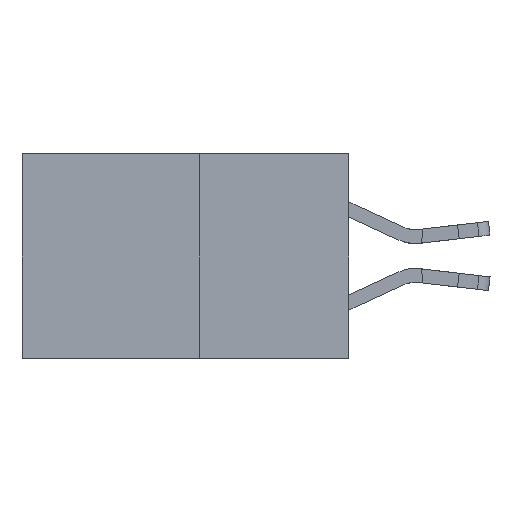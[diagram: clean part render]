
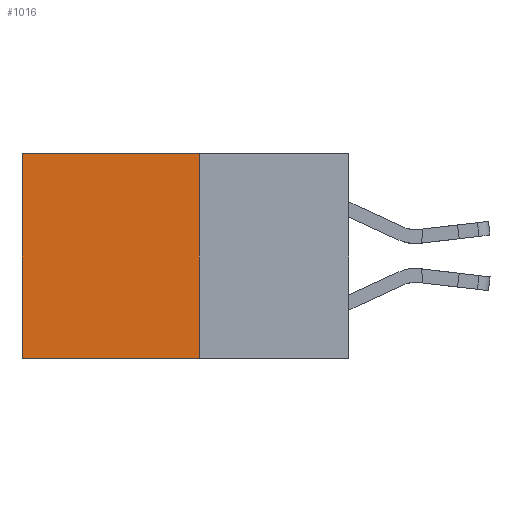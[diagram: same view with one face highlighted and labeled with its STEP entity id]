
A CAD part, left-side view. The second image highlights one B-rep face of the part: STEP entity #1016.
In plain terms, the highlighted planar face has unit normal (-1, 0, 0).
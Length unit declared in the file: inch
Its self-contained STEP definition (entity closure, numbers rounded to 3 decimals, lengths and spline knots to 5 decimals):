
#75 = VERTEX_POINT ( 'NONE', #10894 ) ;
#809 = EDGE_LOOP ( 'NONE', ( #30463, #26506, #1906, #20530 ) ) ;
#1016 = ADVANCED_FACE ( 'NONE', ( #1435 ), #16280, .F. ) ;
#1435 = FACE_OUTER_BOUND ( 'NONE', #809, .T. ) ;
#1906 = ORIENTED_EDGE ( 'NONE', *, *, #9194, .F. ) ;
#3825 = EDGE_CURVE ( 'NONE', #23485, #16942, #8904, .T. ) ;
#4219 = VECTOR ( 'NONE', #25437, 39.37008 ) ;
#5227 = DIRECTION ( 'NONE',  ( 0., 0., -1. ) ) ;
#6414 = AXIS2_PLACEMENT_3D ( 'NONE', #10796, #13680, #19462 ) ;
#8306 = CARTESIAN_POINT ( 'NONE',  ( 0.277, 0.27, -0.37 ) ) ;
#8904 = LINE ( 'NONE', #30610, #9682 ) ;
#9194 = EDGE_CURVE ( 'NONE', #11147, #75, #24392, .T. ) ;
#9682 = VECTOR ( 'NONE', #11408, 39.37008 ) ;
#10059 = LINE ( 'NONE', #8306, #4219 ) ;
#10796 = CARTESIAN_POINT ( 'NONE',  ( 0.277, 0.27, -0.37 ) ) ;
#10894 = CARTESIAN_POINT ( 'NONE',  ( 0.277, 0.27, -0.37 ) ) ;
#11057 = CARTESIAN_POINT ( 'NONE',  ( 0.277, 0.27, 0. ) ) ;
#11147 = VERTEX_POINT ( 'NONE', #11057 ) ;
#11408 = DIRECTION ( 'NONE',  ( 0., 0., -1. ) ) ;
#11733 = EDGE_CURVE ( 'NONE', #75, #16942, #10059, .T. ) ;
#13680 = DIRECTION ( 'NONE',  ( 1., 0., 0. ) ) ;
#16280 = PLANE ( 'NONE',  #6414 ) ;
#16942 = VERTEX_POINT ( 'NONE', #18706 ) ;
#18706 = CARTESIAN_POINT ( 'NONE',  ( 0.277, 0.59, -0.37 ) ) ;
#19462 = DIRECTION ( 'NONE',  ( 0., 0., -1. ) ) ;
#19467 = CARTESIAN_POINT ( 'NONE',  ( 0.277, 0.59, 0. ) ) ;
#20530 = ORIENTED_EDGE ( 'NONE', *, *, #27168, .T. ) ;
#23485 = VERTEX_POINT ( 'NONE', #19467 ) ;
#24392 = LINE ( 'NONE', #29544, #29923 ) ;
#25388 = CARTESIAN_POINT ( 'NONE',  ( 0.277, 0.27, 0. ) ) ;
#25437 = DIRECTION ( 'NONE',  ( 0., 1., 0. ) ) ;
#26506 = ORIENTED_EDGE ( 'NONE', *, *, #11733, .F. ) ;
#27168 = EDGE_CURVE ( 'NONE', #11147, #23485, #29997, .T. ) ;
#27781 = DIRECTION ( 'NONE',  ( 0., 1., 0. ) ) ;
#29275 = VECTOR ( 'NONE', #27781, 39.37008 ) ;
#29544 = CARTESIAN_POINT ( 'NONE',  ( 0.277, 0.27, -0.37 ) ) ;
#29923 = VECTOR ( 'NONE', #5227, 39.37008 ) ;
#29997 = LINE ( 'NONE', #25388, #29275 ) ;
#30463 = ORIENTED_EDGE ( 'NONE', *, *, #3825, .T. ) ;
#30610 = CARTESIAN_POINT ( 'NONE',  ( 0.277, 0.59, -0.37 ) ) ;
